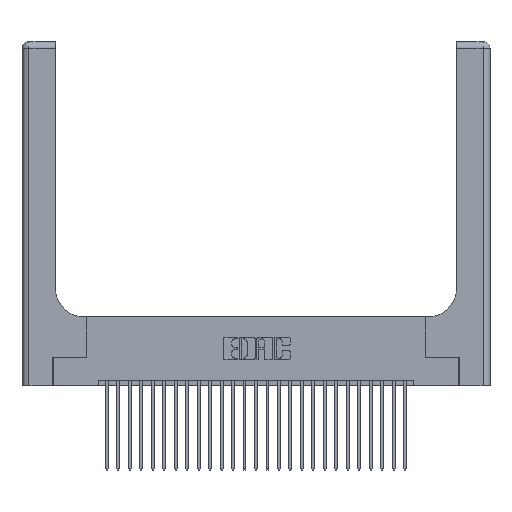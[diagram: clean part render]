
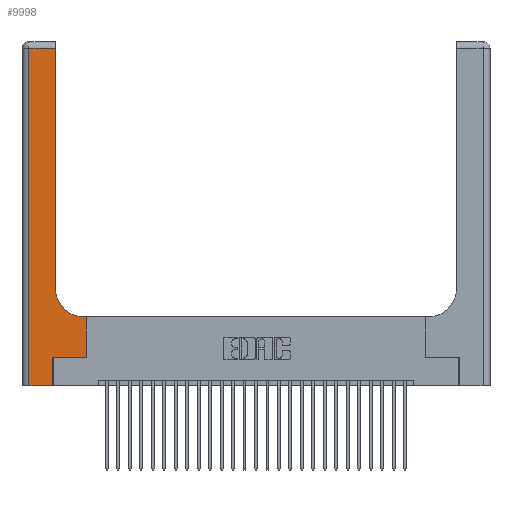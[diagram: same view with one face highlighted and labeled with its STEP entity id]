
A CAD part, top view. The second image highlights one B-rep face of the part: STEP entity #9998.
In plain terms, the highlighted planar face has unit normal (0, 0, 1).
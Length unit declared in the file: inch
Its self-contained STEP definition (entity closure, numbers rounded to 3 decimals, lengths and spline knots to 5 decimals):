
#582 = ORIENTED_EDGE ( 'NONE', *, *, #2925, .T. ) ;
#608 = EDGE_CURVE ( 'NONE', #10370, #25446, #11973, .T. ) ;
#1231 = CARTESIAN_POINT ( 'NONE',  ( 0.06, 0., 0.37 ) ) ;
#1670 = DIRECTION ( 'NONE',  ( 0., -1., 0. ) ) ;
#1727 = AXIS2_PLACEMENT_3D ( 'NONE', #27724, #7898, #12187 ) ;
#2766 = EDGE_LOOP ( 'NONE', ( #16856, #21561, #21639, #6763, #3048, #582, #16441, #26013, #5874 ) ) ;
#2925 = EDGE_CURVE ( 'NONE', #27576, #18684, #7725, .T. ) ;
#3048 = ORIENTED_EDGE ( 'NONE', *, *, #20774, .T. ) ;
#3361 = LINE ( 'NONE', #19893, #22642 ) ;
#4212 = VECTOR ( 'NONE', #11199, 39.37008 ) ;
#4334 = DIRECTION ( 'NONE',  ( 1., 0., 0. ) ) ;
#5003 = CARTESIAN_POINT ( 'NONE',  ( 0.2915, 3., 0.37 ) ) ;
#5450 = LINE ( 'NONE', #5748, #17185 ) ;
#5748 = CARTESIAN_POINT ( 'NONE',  ( 0.269, 0., 0.37 ) ) ;
#5874 = ORIENTED_EDGE ( 'NONE', *, *, #608, .T. ) ;
#5882 = CARTESIAN_POINT ( 'NONE',  ( 0.269, 0.25, 0.37 ) ) ;
#6763 = ORIENTED_EDGE ( 'NONE', *, *, #16859, .T. ) ;
#7113 = EDGE_CURVE ( 'NONE', #25446, #24017, #17698, .T. ) ;
#7725 = LINE ( 'NONE', #10416, #8086 ) ;
#7842 = EDGE_CURVE ( 'NONE', #14711, #10370, #25863, .T. ) ;
#7898 = DIRECTION ( 'NONE',  ( 0., 0., -1. ) ) ;
#7903 = CARTESIAN_POINT ( 'NONE',  ( 0.5415, 0.85, 0.37 ) ) ;
#8086 = VECTOR ( 'NONE', #24064, 39.37008 ) ;
#8603 = FACE_OUTER_BOUND ( 'NONE', #2766, .T. ) ;
#8789 = CARTESIAN_POINT ( 'NONE',  ( 0.2915, 2.94, 0.37 ) ) ;
#8996 = CARTESIAN_POINT ( 'NONE',  ( 0.2915, 0.6, 0.37 ) ) ;
#9998 = ADVANCED_FACE ( 'NONE', ( #8603 ), #12381, .F. ) ;
#10060 = DIRECTION ( 'NONE',  ( 0., 1., 0. ) ) ;
#10370 = VERTEX_POINT ( 'NONE', #11286 ) ;
#10416 = CARTESIAN_POINT ( 'NONE',  ( 0.269, 0.25, 0.37 ) ) ;
#10622 = LINE ( 'NONE', #15103, #26739 ) ;
#11199 = DIRECTION ( 'NONE',  ( -1., 0., 0. ) ) ;
#11286 = CARTESIAN_POINT ( 'NONE',  ( 0.5415, 0.6, 0.37 ) ) ;
#11399 = DIRECTION ( 'NONE',  ( 0., 1., 0. ) ) ;
#11951 = CARTESIAN_POINT ( 'NONE',  ( 0.5585, 0.25, 0.37 ) ) ;
#11973 = CIRCLE ( 'NONE', #15002, 0.25 ) ;
#12187 = DIRECTION ( 'NONE',  ( -1., 0., 0. ) ) ;
#12381 = PLANE ( 'NONE',  #1727 ) ;
#13206 = VECTOR ( 'NONE', #27534, 39.37008 ) ;
#13914 = CARTESIAN_POINT ( 'NONE',  ( 0.2915, 0.85, 0.37 ) ) ;
#13952 = VERTEX_POINT ( 'NONE', #18829 ) ;
#14541 = EDGE_CURVE ( 'NONE', #24017, #13952, #25481, .T. ) ;
#14711 = VERTEX_POINT ( 'NONE', #20420 ) ;
#15002 = AXIS2_PLACEMENT_3D ( 'NONE', #7903, #23272, #21183 ) ;
#15103 = CARTESIAN_POINT ( 'NONE',  ( 0., 0., 0.37 ) ) ;
#16441 = ORIENTED_EDGE ( 'NONE', *, *, #17737, .T. ) ;
#16458 = LINE ( 'NONE', #21280, #23305 ) ;
#16608 = DIRECTION ( 'NONE',  ( -1., 0., 0. ) ) ;
#16856 = ORIENTED_EDGE ( 'NONE', *, *, #7113, .T. ) ;
#16859 = EDGE_CURVE ( 'NONE', #20594, #23411, #10622, .T. ) ;
#17185 = VECTOR ( 'NONE', #10060, 39.37008 ) ;
#17698 = LINE ( 'NONE', #5003, #13206 ) ;
#17737 = EDGE_CURVE ( 'NONE', #18684, #14711, #3361, .T. ) ;
#18684 = VERTEX_POINT ( 'NONE', #11951 ) ;
#18829 = CARTESIAN_POINT ( 'NONE',  ( 0.06, 2.94, 0.37 ) ) ;
#18978 = VECTOR ( 'NONE', #16608, 39.37008 ) ;
#19893 = CARTESIAN_POINT ( 'NONE',  ( 0.5585, 0.25, 0.37 ) ) ;
#20420 = CARTESIAN_POINT ( 'NONE',  ( 0.5585, 0.6, 0.37 ) ) ;
#20594 = VERTEX_POINT ( 'NONE', #1231 ) ;
#20774 = EDGE_CURVE ( 'NONE', #23411, #27576, #5450, .T. ) ;
#21030 = CARTESIAN_POINT ( 'NONE',  ( 0., 2.94, 0.37 ) ) ;
#21183 = DIRECTION ( 'NONE',  ( 1., 0., 0. ) ) ;
#21280 = CARTESIAN_POINT ( 'NONE',  ( 0.06, 3., 0.37 ) ) ;
#21561 = ORIENTED_EDGE ( 'NONE', *, *, #14541, .T. ) ;
#21639 = ORIENTED_EDGE ( 'NONE', *, *, #21897, .T. ) ;
#21897 = EDGE_CURVE ( 'NONE', #13952, #20594, #16458, .T. ) ;
#22642 = VECTOR ( 'NONE', #11399, 39.37008 ) ;
#23272 = DIRECTION ( 'NONE',  ( 0., 0., -1. ) ) ;
#23305 = VECTOR ( 'NONE', #1670, 39.37008 ) ;
#23411 = VERTEX_POINT ( 'NONE', #25191 ) ;
#24017 = VERTEX_POINT ( 'NONE', #8789 ) ;
#24064 = DIRECTION ( 'NONE',  ( 1., 0., 0. ) ) ;
#25191 = CARTESIAN_POINT ( 'NONE',  ( 0.269, 0., 0.37 ) ) ;
#25446 = VERTEX_POINT ( 'NONE', #13914 ) ;
#25481 = LINE ( 'NONE', #21030, #18978 ) ;
#25863 = LINE ( 'NONE', #8996, #4212 ) ;
#26013 = ORIENTED_EDGE ( 'NONE', *, *, #7842, .T. ) ;
#26739 = VECTOR ( 'NONE', #4334, 39.37008 ) ;
#27534 = DIRECTION ( 'NONE',  ( 0., 1., 0. ) ) ;
#27576 = VERTEX_POINT ( 'NONE', #5882 ) ;
#27724 = CARTESIAN_POINT ( 'NONE',  ( 0., 3., 0.37 ) ) ;
